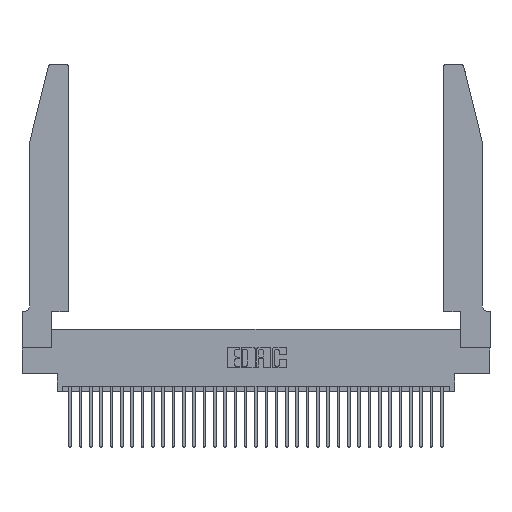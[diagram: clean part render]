
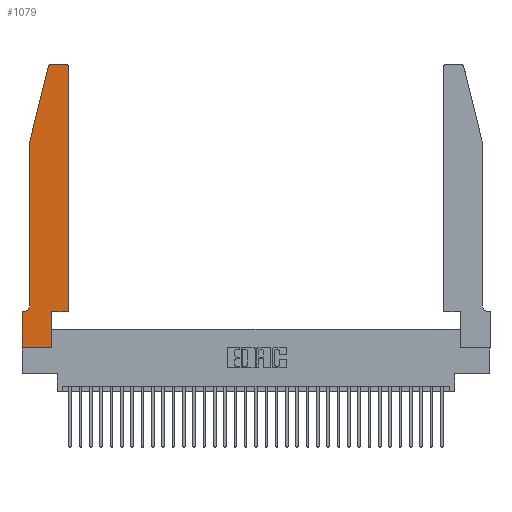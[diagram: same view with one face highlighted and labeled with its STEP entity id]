
A CAD part, top view. The second image highlights one B-rep face of the part: STEP entity #1079.
In plain terms, the highlighted planar face has unit normal (0, 0, 1).
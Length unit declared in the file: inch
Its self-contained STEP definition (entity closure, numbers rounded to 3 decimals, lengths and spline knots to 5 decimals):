
#142 = CARTESIAN_POINT ( 'NONE',  ( 0.0055, 0.42, 0.37 ) ) ;
#468 = LINE ( 'NONE', #18444, #14149 ) ;
#602 = DIRECTION ( 'NONE',  ( 0., -1., 0. ) ) ;
#1079 = ADVANCED_FACE ( 'NONE', ( #24854 ), #21188, .T. ) ;
#1895 = DIRECTION ( 'NONE',  ( 1., 0., 0. ) ) ;
#2059 = CIRCLE ( 'NONE', #8501, 0.03 ) ;
#2572 = EDGE_CURVE ( 'NONE', #29564, #33003, #25588, .T. ) ;
#2932 = DIRECTION ( 'NONE',  ( -1., 0., 0. ) ) ;
#3106 = CARTESIAN_POINT ( 'NONE',  ( 0.0755, 2., 0.37 ) ) ;
#3385 = VERTEX_POINT ( 'NONE', #30125 ) ;
#3389 = VERTEX_POINT ( 'NONE', #30011 ) ;
#3422 = EDGE_CURVE ( 'NONE', #3389, #29123, #22273, .T. ) ;
#3947 = CARTESIAN_POINT ( 'NONE',  ( 0.25487, 2.72718, 0.37 ) ) ;
#4029 = ORIENTED_EDGE ( 'NONE', *, *, #2572, .T. ) ;
#4463 = ORIENTED_EDGE ( 'NONE', *, *, #21375, .T. ) ;
#4599 = CARTESIAN_POINT ( 'NONE',  ( 0.2605, 2.75, 0.37 ) ) ;
#4663 = CARTESIAN_POINT ( 'NONE',  ( 0.2865, 0.35, 0.37 ) ) ;
#5641 = VERTEX_POINT ( 'NONE', #21157 ) ;
#6279 = CARTESIAN_POINT ( 'NONE',  ( 0.0755, 0.42, 0.37 ) ) ;
#6771 = VERTEX_POINT ( 'NONE', #4663 ) ;
#7014 = ORIENTED_EDGE ( 'NONE', *, *, #16656, .T. ) ;
#7032 = DIRECTION ( 'NONE',  ( 0., -1., 0. ) ) ;
#7141 = CARTESIAN_POINT ( 'NONE',  ( 0.2865, 0.35, 0.37 ) ) ;
#7251 = VECTOR ( 'NONE', #23430, 39.37008 ) ;
#7390 = EDGE_CURVE ( 'NONE', #29123, #6771, #24220, .T. ) ;
#7499 = AXIS2_PLACEMENT_3D ( 'NONE', #24008, #31976, #1895 ) ;
#7754 = CARTESIAN_POINT ( 'NONE',  ( 0.284, 2.72, 0.37 ) ) ;
#7905 = ORIENTED_EDGE ( 'NONE', *, *, #22954, .T. ) ;
#7950 = DIRECTION ( 'NONE',  ( 0., 1., 0. ) ) ;
#8308 = ORIENTED_EDGE ( 'NONE', *, *, #3422, .T. ) ;
#8501 = AXIS2_PLACEMENT_3D ( 'NONE', #7754, #26453, #10472 ) ;
#9079 = LINE ( 'NONE', #27805, #28649 ) ;
#9624 = DIRECTION ( 'NONE',  ( 0., 0., 1. ) ) ;
#10004 = ORIENTED_EDGE ( 'NONE', *, *, #24630, .T. ) ;
#10472 = DIRECTION ( 'NONE',  ( 1., 0., 0. ) ) ;
#10766 = VERTEX_POINT ( 'NONE', #16008 ) ;
#11265 = ORIENTED_EDGE ( 'NONE', *, *, #27787, .T. ) ;
#11454 = LINE ( 'NONE', #32002, #17757 ) ;
#12644 = EDGE_LOOP ( 'NONE', ( #18652, #23008, #22174, #7905, #4463, #32023, #10004, #8308, #32397, #11265, #4029, #7014 ) ) ;
#13547 = LINE ( 'NONE', #32659, #26832 ) ;
#14149 = VECTOR ( 'NONE', #21146, 39.37008 ) ;
#14445 = LINE ( 'NONE', #4599, #7251 ) ;
#14453 = CARTESIAN_POINT ( 'NONE',  ( 0.0055, 0.35, 0.37 ) ) ;
#14944 = EDGE_CURVE ( 'NONE', #18952, #5641, #14445, .T. ) ;
#15308 = DIRECTION ( 'NONE',  ( 0., 1., 0. ) ) ;
#16006 = CARTESIAN_POINT ( 'NONE',  ( 0.4505, 0.35, 0.37 ) ) ;
#16008 = CARTESIAN_POINT ( 'NONE',  ( 0.0755, 2., 0.37 ) ) ;
#16211 = DIRECTION ( 'NONE',  ( -1., 0., 0. ) ) ;
#16656 = EDGE_CURVE ( 'NONE', #33003, #18952, #24726, .T. ) ;
#17757 = VECTOR ( 'NONE', #16211, 39.37008 ) ;
#18444 = CARTESIAN_POINT ( 'NONE',  ( 0.4505, 0.35, 0.37 ) ) ;
#18652 = ORIENTED_EDGE ( 'NONE', *, *, #14944, .T. ) ;
#18901 = EDGE_CURVE ( 'NONE', #5641, #34409, #2059, .T. ) ;
#18952 = VERTEX_POINT ( 'NONE', #31831 ) ;
#19094 = VECTOR ( 'NONE', #21970, 39.37008 ) ;
#19135 = DIRECTION ( 'NONE',  ( 0., 0., -1. ) ) ;
#19685 = DIRECTION ( 'NONE',  ( 1., 0., 0. ) ) ;
#21146 = DIRECTION ( 'NONE',  ( 1., 0., 0. ) ) ;
#21157 = CARTESIAN_POINT ( 'NONE',  ( 0.284, 2.75, 0.37 ) ) ;
#21188 = PLANE ( 'NONE',  #7499 ) ;
#21375 = EDGE_CURVE ( 'NONE', #28743, #32558, #29139, .T. ) ;
#21474 = VECTOR ( 'NONE', #19685, 39.37008 ) ;
#21741 = VECTOR ( 'NONE', #15308, 39.37008 ) ;
#21970 = DIRECTION ( 'NONE',  ( -0.239, -0.971, 0. ) ) ;
#22174 = ORIENTED_EDGE ( 'NONE', *, *, #31793, .T. ) ;
#22273 = LINE ( 'NONE', #22443, #21474 ) ;
#22443 = CARTESIAN_POINT ( 'NONE',  ( 0., 0., 0.37 ) ) ;
#22466 = AXIS2_PLACEMENT_3D ( 'NONE', #142, #19135, #2932 ) ;
#22954 = EDGE_CURVE ( 'NONE', #10766, #28743, #9079, .T. ) ;
#23008 = ORIENTED_EDGE ( 'NONE', *, *, #18901, .T. ) ;
#23430 = DIRECTION ( 'NONE',  ( -1., 0., 0. ) ) ;
#23461 = CARTESIAN_POINT ( 'NONE',  ( 0.4505, 0.35, 0.37 ) ) ;
#24008 = CARTESIAN_POINT ( 'NONE',  ( 0., 0.35, 0.37 ) ) ;
#24220 = LINE ( 'NONE', #7141, #21741 ) ;
#24630 = EDGE_CURVE ( 'NONE', #3385, #3389, #13547, .T. ) ;
#24726 = CIRCLE ( 'NONE', #32914, 0.03 ) ;
#24758 = VECTOR ( 'NONE', #7950, 39.37008 ) ;
#24854 = FACE_OUTER_BOUND ( 'NONE', #12644, .T. ) ;
#25588 = LINE ( 'NONE', #16006, #24758 ) ;
#25621 = CARTESIAN_POINT ( 'NONE',  ( 0.4205, 2.72, 0.37 ) ) ;
#26122 = LINE ( 'NONE', #3106, #19094 ) ;
#26453 = DIRECTION ( 'NONE',  ( 0., 0., 1. ) ) ;
#26830 = CARTESIAN_POINT ( 'NONE',  ( 0.2865, 0., 0.37 ) ) ;
#26832 = VECTOR ( 'NONE', #602, 39.37008 ) ;
#27787 = EDGE_CURVE ( 'NONE', #6771, #29564, #468, .T. ) ;
#27805 = CARTESIAN_POINT ( 'NONE',  ( 0.0755, 2., 0.37 ) ) ;
#28253 = DIRECTION ( 'NONE',  ( 1., 0., 0. ) ) ;
#28649 = VECTOR ( 'NONE', #7032, 39.37008 ) ;
#28743 = VERTEX_POINT ( 'NONE', #6279 ) ;
#29123 = VERTEX_POINT ( 'NONE', #26830 ) ;
#29139 = CIRCLE ( 'NONE', #22466, 0.07 ) ;
#29564 = VERTEX_POINT ( 'NONE', #23461 ) ;
#30011 = CARTESIAN_POINT ( 'NONE',  ( 0., 0., 0.37 ) ) ;
#30125 = CARTESIAN_POINT ( 'NONE',  ( 0., 0.35, 0.37 ) ) ;
#31793 = EDGE_CURVE ( 'NONE', #34409, #10766, #26122, .T. ) ;
#31831 = CARTESIAN_POINT ( 'NONE',  ( 0.4205, 2.75, 0.37 ) ) ;
#31976 = DIRECTION ( 'NONE',  ( 0., 0., 1. ) ) ;
#32002 = CARTESIAN_POINT ( 'NONE',  ( 0.0755, 0.35, 0.37 ) ) ;
#32023 = ORIENTED_EDGE ( 'NONE', *, *, #32982, .T. ) ;
#32099 = CARTESIAN_POINT ( 'NONE',  ( 0.4505, 2.72, 0.37 ) ) ;
#32397 = ORIENTED_EDGE ( 'NONE', *, *, #7390, .T. ) ;
#32558 = VERTEX_POINT ( 'NONE', #14453 ) ;
#32659 = CARTESIAN_POINT ( 'NONE',  ( 0., 0., 0.37 ) ) ;
#32914 = AXIS2_PLACEMENT_3D ( 'NONE', #25621, #9624, #28253 ) ;
#32982 = EDGE_CURVE ( 'NONE', #32558, #3385, #11454, .T. ) ;
#33003 = VERTEX_POINT ( 'NONE', #32099 ) ;
#34409 = VERTEX_POINT ( 'NONE', #3947 ) ;
